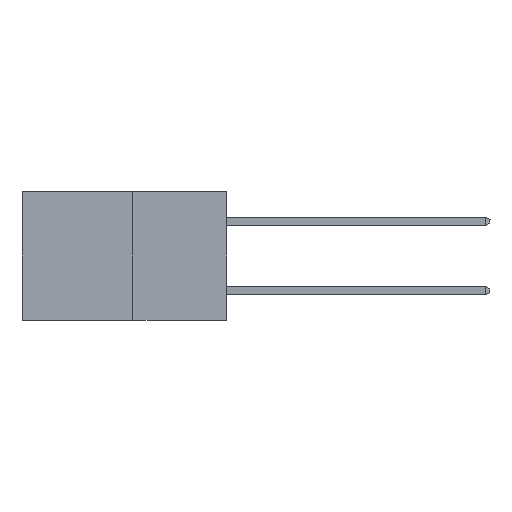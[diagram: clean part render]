
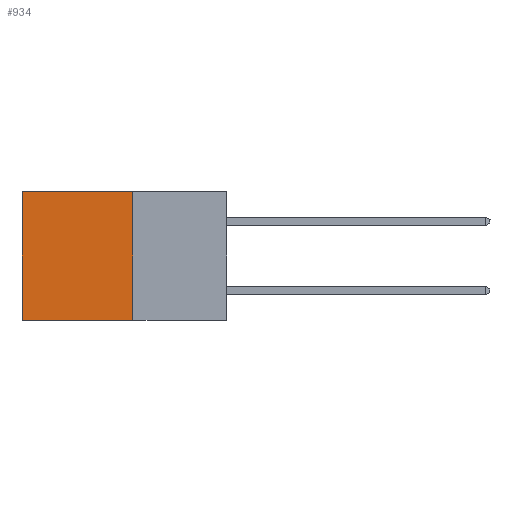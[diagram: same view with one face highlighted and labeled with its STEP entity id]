
A CAD part, left-side view. The second image highlights one B-rep face of the part: STEP entity #934.
In plain terms, the highlighted planar face has unit normal (-1, 0, 0).
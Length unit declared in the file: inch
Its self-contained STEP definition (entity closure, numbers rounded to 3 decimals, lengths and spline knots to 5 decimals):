
#64 = EDGE_LOOP ( 'NONE', ( #9031, #13477, #17298, #13961 ) ) ;
#934 = ADVANCED_FACE ( 'NONE', ( #14070 ), #3662, .F. ) ;
#1310 = LINE ( 'NONE', #11277, #16702 ) ;
#1741 = VECTOR ( 'NONE', #12661, 39.37008 ) ;
#2349 = VERTEX_POINT ( 'NONE', #10699 ) ;
#2719 = CARTESIAN_POINT ( 'NONE',  ( 0.277, 0.27, 0. ) ) ;
#3639 = DIRECTION ( 'NONE',  ( 1., 0., 0. ) ) ;
#3662 = PLANE ( 'NONE',  #10289 ) ;
#4135 = VECTOR ( 'NONE', #6819, 39.37008 ) ;
#4194 = DIRECTION ( 'NONE',  ( 0., 1., 0. ) ) ;
#5069 = CARTESIAN_POINT ( 'NONE',  ( 0.277, 0.59, 0. ) ) ;
#5778 = LINE ( 'NONE', #12518, #1741 ) ;
#6211 = VECTOR ( 'NONE', #4194, 39.37008 ) ;
#6473 = VERTEX_POINT ( 'NONE', #5069 ) ;
#6819 = DIRECTION ( 'NONE',  ( 0., 0., -1. ) ) ;
#7732 = EDGE_CURVE ( 'NONE', #16883, #14923, #5778, .T. ) ;
#8500 = CARTESIAN_POINT ( 'NONE',  ( 0.277, 0.27, -0.37 ) ) ;
#9031 = ORIENTED_EDGE ( 'NONE', *, *, #12574, .T. ) ;
#9776 = CARTESIAN_POINT ( 'NONE',  ( 0.277, 0.27, -0.37 ) ) ;
#10197 = LINE ( 'NONE', #2719, #6211 ) ;
#10289 = AXIS2_PLACEMENT_3D ( 'NONE', #8500, #3639, #13352 ) ;
#10498 = CARTESIAN_POINT ( 'NONE',  ( 0.277, 0.59, -0.37 ) ) ;
#10699 = CARTESIAN_POINT ( 'NONE',  ( 0.277, 0.27, 0. ) ) ;
#11277 = CARTESIAN_POINT ( 'NONE',  ( 0.277, 0.59, -0.37 ) ) ;
#12518 = CARTESIAN_POINT ( 'NONE',  ( 0.277, 0.27, -0.37 ) ) ;
#12574 = EDGE_CURVE ( 'NONE', #6473, #14923, #1310, .T. ) ;
#12651 = LINE ( 'NONE', #9776, #4135 ) ;
#12661 = DIRECTION ( 'NONE',  ( 0., 1., 0. ) ) ;
#13352 = DIRECTION ( 'NONE',  ( 0., 0., -1. ) ) ;
#13477 = ORIENTED_EDGE ( 'NONE', *, *, #7732, .F. ) ;
#13961 = ORIENTED_EDGE ( 'NONE', *, *, #15744, .T. ) ;
#14070 = FACE_OUTER_BOUND ( 'NONE', #64, .T. ) ;
#14439 = CARTESIAN_POINT ( 'NONE',  ( 0.277, 0.27, -0.37 ) ) ;
#14923 = VERTEX_POINT ( 'NONE', #10498 ) ;
#15704 = DIRECTION ( 'NONE',  ( 0., 0., -1. ) ) ;
#15744 = EDGE_CURVE ( 'NONE', #2349, #6473, #10197, .T. ) ;
#16702 = VECTOR ( 'NONE', #15704, 39.37008 ) ;
#16883 = VERTEX_POINT ( 'NONE', #14439 ) ;
#17298 = ORIENTED_EDGE ( 'NONE', *, *, #18206, .F. ) ;
#18206 = EDGE_CURVE ( 'NONE', #2349, #16883, #12651, .T. ) ;
